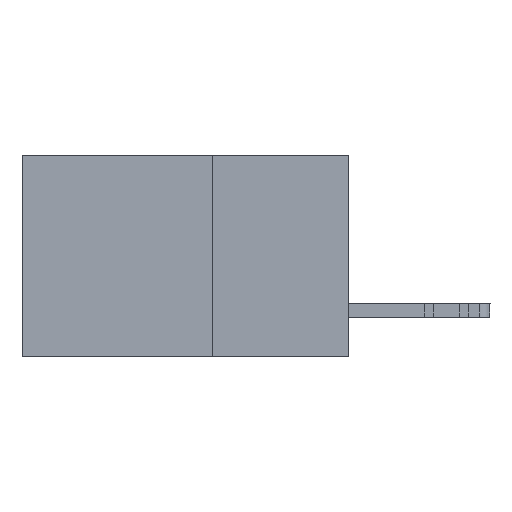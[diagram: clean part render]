
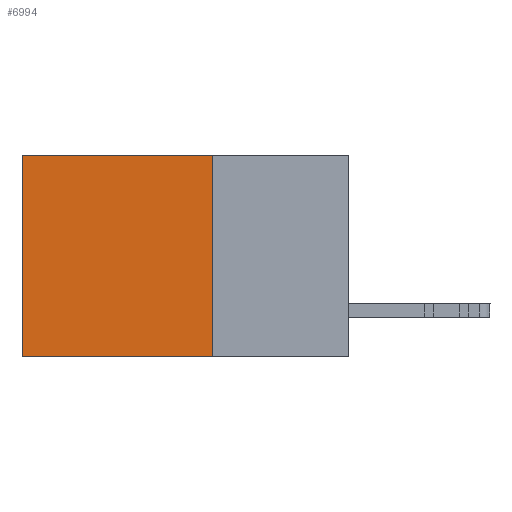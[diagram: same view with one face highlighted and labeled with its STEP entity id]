
A CAD part, left-side view. The second image highlights one B-rep face of the part: STEP entity #6994.
In plain terms, the highlighted planar face has unit normal (-1, 0, 0).
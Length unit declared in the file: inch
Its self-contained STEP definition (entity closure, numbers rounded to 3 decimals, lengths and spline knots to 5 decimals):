
#176 = CARTESIAN_POINT ( 'NONE',  ( 0.2615, 0.25, 0. ) ) ;
#749 = ORIENTED_EDGE ( 'NONE', *, *, #23640, .F. ) ;
#2550 = ORIENTED_EDGE ( 'NONE', *, *, #22848, .T. ) ;
#2839 = EDGE_CURVE ( 'NONE', #6888, #8262, #15337, .T. ) ;
#3469 = CARTESIAN_POINT ( 'NONE',  ( 0.2615, 0.6, 0. ) ) ;
#3851 = LINE ( 'NONE', #176, #7557 ) ;
#4933 = DIRECTION ( 'NONE',  ( 0., 0., -1. ) ) ;
#6888 = VERTEX_POINT ( 'NONE', #19132 ) ;
#6889 = EDGE_LOOP ( 'NONE', ( #18731, #749, #10976, #2550 ) ) ;
#6994 = ADVANCED_FACE ( 'NONE', ( #13640 ), #15725, .F. ) ;
#7557 = VECTOR ( 'NONE', #22684, 39.37008 ) ;
#7611 = CARTESIAN_POINT ( 'NONE',  ( 0.2615, 0.25, -0.37 ) ) ;
#7742 = VECTOR ( 'NONE', #16683, 39.37008 ) ;
#7751 = AXIS2_PLACEMENT_3D ( 'NONE', #21324, #23282, #4933 ) ;
#8262 = VERTEX_POINT ( 'NONE', #13523 ) ;
#9162 = CARTESIAN_POINT ( 'NONE',  ( 0.2615, 0.6, -0.37 ) ) ;
#9600 = DIRECTION ( 'NONE',  ( 0., 1., 0. ) ) ;
#9723 = VERTEX_POINT ( 'NONE', #3469 ) ;
#10624 = VECTOR ( 'NONE', #23601, 39.37008 ) ;
#10976 = ORIENTED_EDGE ( 'NONE', *, *, #2839, .F. ) ;
#13523 = CARTESIAN_POINT ( 'NONE',  ( 0.2615, 0.25, -0.37 ) ) ;
#13640 = FACE_OUTER_BOUND ( 'NONE', #6889, .T. ) ;
#15337 = LINE ( 'NONE', #7611, #7742 ) ;
#15725 = PLANE ( 'NONE',  #7751 ) ;
#16521 = LINE ( 'NONE', #9162, #10624 ) ;
#16568 = VECTOR ( 'NONE', #9600, 39.37008 ) ;
#16683 = DIRECTION ( 'NONE',  ( 0., 0., -1. ) ) ;
#17475 = CARTESIAN_POINT ( 'NONE',  ( 0.2615, 0.6, -0.37 ) ) ;
#18731 = ORIENTED_EDGE ( 'NONE', *, *, #20604, .T. ) ;
#18901 = LINE ( 'NONE', #22808, #16568 ) ;
#19132 = CARTESIAN_POINT ( 'NONE',  ( 0.2615, 0.25, 0. ) ) ;
#20604 = EDGE_CURVE ( 'NONE', #9723, #21000, #16521, .T. ) ;
#21000 = VERTEX_POINT ( 'NONE', #17475 ) ;
#21324 = CARTESIAN_POINT ( 'NONE',  ( 0.2615, 0.25, -0.37 ) ) ;
#22684 = DIRECTION ( 'NONE',  ( 0., 1., 0. ) ) ;
#22808 = CARTESIAN_POINT ( 'NONE',  ( 0.2615, 0.25, -0.37 ) ) ;
#22848 = EDGE_CURVE ( 'NONE', #6888, #9723, #3851, .T. ) ;
#23282 = DIRECTION ( 'NONE',  ( 1., 0., 0. ) ) ;
#23601 = DIRECTION ( 'NONE',  ( 0., 0., -1. ) ) ;
#23640 = EDGE_CURVE ( 'NONE', #8262, #21000, #18901, .T. ) ;
